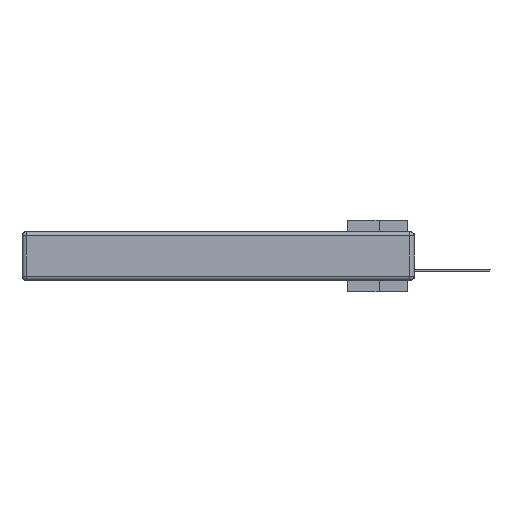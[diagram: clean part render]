
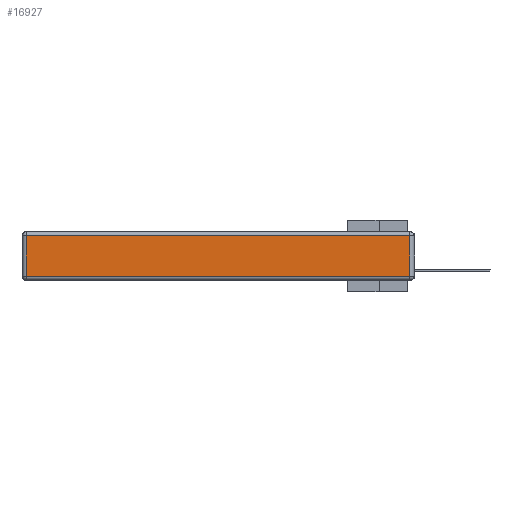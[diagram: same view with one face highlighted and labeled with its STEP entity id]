
A CAD part, left-side view. The second image highlights one B-rep face of the part: STEP entity #16927.
In plain terms, the highlighted planar face has unit normal (-1, 0, 0).
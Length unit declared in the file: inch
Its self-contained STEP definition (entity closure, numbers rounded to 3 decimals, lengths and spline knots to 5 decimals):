
#323 = VECTOR ( 'NONE', #25485, 39.37008 ) ;
#1786 = DIRECTION ( 'NONE',  ( 0., 0., 1. ) ) ;
#2346 = AXIS2_PLACEMENT_3D ( 'NONE', #23280, #23111, #1786 ) ;
#2960 = VECTOR ( 'NONE', #13355, 39.37008 ) ;
#3834 = EDGE_CURVE ( 'NONE', #14591, #23845, #11011, .T. ) ;
#5574 = DIRECTION ( 'NONE',  ( 0., -1., 0. ) ) ;
#5963 = ORIENTED_EDGE ( 'NONE', *, *, #21122, .T. ) ;
#7653 = CARTESIAN_POINT ( 'NONE',  ( 0., 2.72, -0.343 ) ) ;
#10189 = LINE ( 'NONE', #7653, #323 ) ;
#11011 = LINE ( 'NONE', #11355, #16266 ) ;
#11355 = CARTESIAN_POINT ( 'NONE',  ( 0., 0., -0.313 ) ) ;
#12686 = CARTESIAN_POINT ( 'NONE',  ( 0., 2.75, -0.03 ) ) ;
#12749 = FACE_OUTER_BOUND ( 'NONE', #19827, .T. ) ;
#13121 = LINE ( 'NONE', #20951, #18280 ) ;
#13355 = DIRECTION ( 'NONE',  ( 0., 1., 0. ) ) ;
#13774 = ORIENTED_EDGE ( 'NONE', *, *, #3834, .T. ) ;
#14591 = VERTEX_POINT ( 'NONE', #26808 ) ;
#16266 = VECTOR ( 'NONE', #5574, 39.37008 ) ;
#16386 = CARTESIAN_POINT ( 'NONE',  ( 0., 0.03, -0.313 ) ) ;
#16927 = ADVANCED_FACE ( 'NONE', ( #12749 ), #25814, .T. ) ;
#18280 = VECTOR ( 'NONE', #20785, 39.37008 ) ;
#18680 = EDGE_CURVE ( 'NONE', #23932, #22416, #30867, .T. ) ;
#19066 = ORIENTED_EDGE ( 'NONE', *, *, #21935, .T. ) ;
#19827 = EDGE_LOOP ( 'NONE', ( #13774, #19066, #29291, #5963 ) ) ;
#20785 = DIRECTION ( 'NONE',  ( 0., 0., 1. ) ) ;
#20951 = CARTESIAN_POINT ( 'NONE',  ( 0., 0.03, -0.343 ) ) ;
#21122 = EDGE_CURVE ( 'NONE', #22416, #14591, #10189, .T. ) ;
#21935 = EDGE_CURVE ( 'NONE', #23845, #23932, #13121, .T. ) ;
#22163 = CARTESIAN_POINT ( 'NONE',  ( 0., 0.03, -0.03 ) ) ;
#22416 = VERTEX_POINT ( 'NONE', #25651 ) ;
#23111 = DIRECTION ( 'NONE',  ( -1., 0., 0. ) ) ;
#23280 = CARTESIAN_POINT ( 'NONE',  ( 0., 0., -0.343 ) ) ;
#23845 = VERTEX_POINT ( 'NONE', #16386 ) ;
#23932 = VERTEX_POINT ( 'NONE', #22163 ) ;
#25485 = DIRECTION ( 'NONE',  ( 0., 0., -1. ) ) ;
#25651 = CARTESIAN_POINT ( 'NONE',  ( 0., 2.72, -0.03 ) ) ;
#25814 = PLANE ( 'NONE',  #2346 ) ;
#26808 = CARTESIAN_POINT ( 'NONE',  ( 0., 2.72, -0.313 ) ) ;
#29291 = ORIENTED_EDGE ( 'NONE', *, *, #18680, .T. ) ;
#30867 = LINE ( 'NONE', #12686, #2960 ) ;
